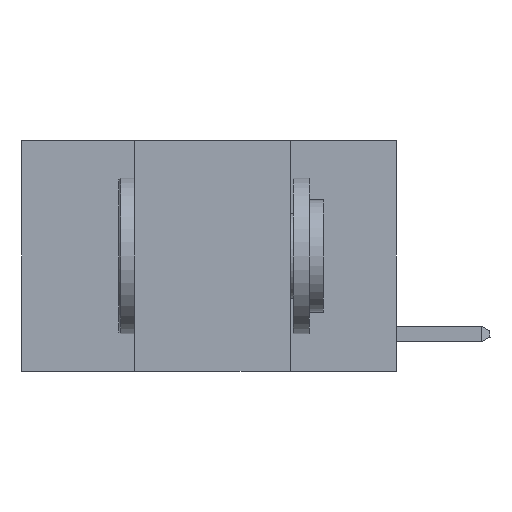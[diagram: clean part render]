
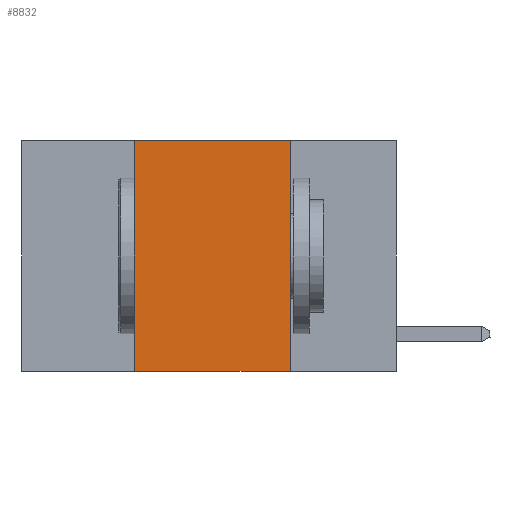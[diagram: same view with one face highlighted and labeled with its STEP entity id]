
A CAD part, left-side view. The second image highlights one B-rep face of the part: STEP entity #8832.
In plain terms, the highlighted planar face has unit normal (-1, 0, 0).
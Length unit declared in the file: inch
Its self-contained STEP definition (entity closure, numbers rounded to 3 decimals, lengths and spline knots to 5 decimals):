
#256 = DIRECTION ( 'NONE',  ( 0., -1., 0. ) ) ;
#314 = LINE ( 'NONE', #3502, #444 ) ;
#363 = EDGE_LOOP ( 'NONE', ( #984, #3664, #4222, #6650 ) ) ;
#382 = EDGE_CURVE ( 'NONE', #2333, #3474, #9353, .T. ) ;
#444 = VECTOR ( 'NONE', #256, 39.37008 ) ;
#825 = DIRECTION ( 'NONE',  ( 1., 0., 0. ) ) ;
#984 = ORIENTED_EDGE ( 'NONE', *, *, #382, .F. ) ;
#1012 = CARTESIAN_POINT ( 'NONE',  ( 0., 0.42, 0. ) ) ;
#1522 = VECTOR ( 'NONE', #7366, 39.37008 ) ;
#1940 = CARTESIAN_POINT ( 'NONE',  ( 0., 0.6, -0.37 ) ) ;
#2068 = CARTESIAN_POINT ( 'NONE',  ( 0., 0.17, 0. ) ) ;
#2165 = CARTESIAN_POINT ( 'NONE',  ( 0., 0.42, -0.37 ) ) ;
#2333 = VERTEX_POINT ( 'NONE', #6240 ) ;
#2540 = CARTESIAN_POINT ( 'NONE',  ( 0., 0.17, -0.37 ) ) ;
#2570 = EDGE_CURVE ( 'NONE', #5391, #3474, #3380, .T. ) ;
#3305 = DIRECTION ( 'NONE',  ( 0., 0., -1. ) ) ;
#3380 = LINE ( 'NONE', #1940, #1522 ) ;
#3386 = VECTOR ( 'NONE', #9133, 39.37008 ) ;
#3474 = VERTEX_POINT ( 'NONE', #2540 ) ;
#3502 = CARTESIAN_POINT ( 'NONE',  ( 0., 0.6, 0. ) ) ;
#3563 = VECTOR ( 'NONE', #8604, 39.37008 ) ;
#3664 = ORIENTED_EDGE ( 'NONE', *, *, #9622, .F. ) ;
#3864 = FACE_OUTER_BOUND ( 'NONE', #363, .T. ) ;
#4222 = ORIENTED_EDGE ( 'NONE', *, *, #6878, .F. ) ;
#5026 = LINE ( 'NONE', #1012, #3386 ) ;
#5391 = VERTEX_POINT ( 'NONE', #2165 ) ;
#6240 = CARTESIAN_POINT ( 'NONE',  ( 0., 0.17, 0. ) ) ;
#6650 = ORIENTED_EDGE ( 'NONE', *, *, #2570, .T. ) ;
#6878 = EDGE_CURVE ( 'NONE', #5391, #8206, #5026, .T. ) ;
#6954 = AXIS2_PLACEMENT_3D ( 'NONE', #7176, #825, #3305 ) ;
#7176 = CARTESIAN_POINT ( 'NONE',  ( 0., 0.6, 0. ) ) ;
#7366 = DIRECTION ( 'NONE',  ( 0., -1., 0. ) ) ;
#7726 = CARTESIAN_POINT ( 'NONE',  ( 0., 0.42, 0. ) ) ;
#8206 = VERTEX_POINT ( 'NONE', #7726 ) ;
#8604 = DIRECTION ( 'NONE',  ( 0., 0., -1. ) ) ;
#8832 = ADVANCED_FACE ( 'NONE', ( #3864 ), #8851, .F. ) ;
#8851 = PLANE ( 'NONE',  #6954 ) ;
#9133 = DIRECTION ( 'NONE',  ( 0., 0., 1. ) ) ;
#9353 = LINE ( 'NONE', #2068, #3563 ) ;
#9622 = EDGE_CURVE ( 'NONE', #8206, #2333, #314, .T. ) ;
